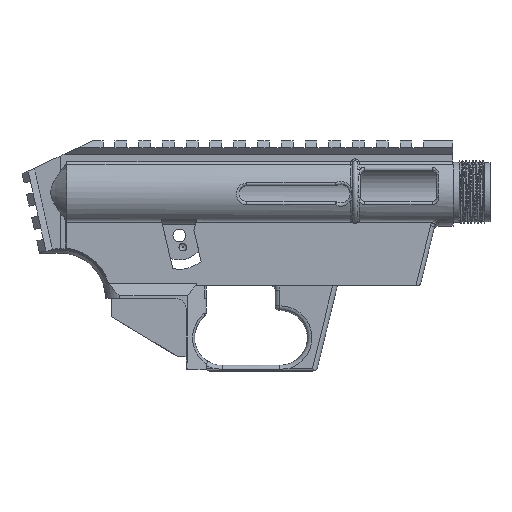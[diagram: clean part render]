
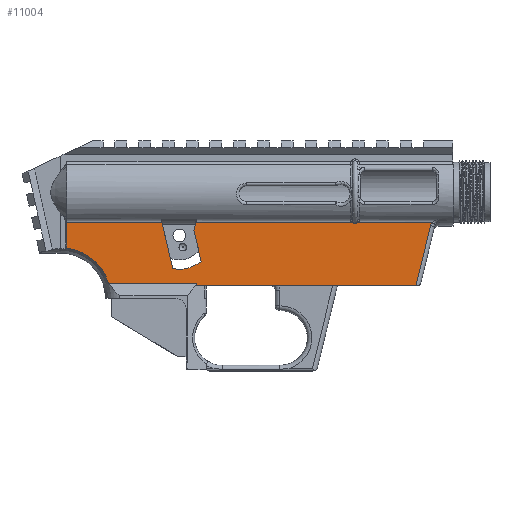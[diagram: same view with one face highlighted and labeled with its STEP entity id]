
A CAD part, left-side view. The second image highlights one B-rep face of the part: STEP entity #11004.
In plain terms, the highlighted planar face has unit normal (-1, 0, 0).
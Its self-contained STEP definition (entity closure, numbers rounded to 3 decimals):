
#329=B_SPLINE_CURVE_WITH_KNOTS('',3,(#16165,#16166,#16167,#16168,#16169,
#16170),.UNSPECIFIED.,.F.,.F.,(4,2,4),(0.,0.074,0.148),
 .UNSPECIFIED.);
#394=B_SPLINE_CURVE_WITH_KNOTS('',3,(#18997,#18998,#18999,#19000,#19001,
#19002,#19003,#19004,#19005,#19006,#19007,#19008),.UNSPECIFIED.,.F.,.F.,
(4,2,2,2,2,4),(0.,0.021,0.047,0.063,
0.077,0.097),.UNSPECIFIED.);
#395=B_SPLINE_CURVE_WITH_KNOTS('',3,(#19010,#19011,#19012,#19013,#19014,
#19015,#19016,#19017,#19018,#19019,#19020,#19021,#19022),.UNSPECIFIED.,
 .F.,.F.,(4,2,2,3,2,4),(-0.102,-0.09,-0.043,
0.,0.045,0.072),.UNSPECIFIED.);
#593=CIRCLE('',#11296,14.884);
#682=CIRCLE('',#11611,22.405);
#1240=FACE_OUTER_BOUND('',#1842,.T.);
#1842=EDGE_LOOP('',(#9356,#9357,#9358,#9359,#9360,#9361,#9362,#9363,#9364,
#9365,#9366,#9367,#9368,#9369,#9370,#9371));
#2151=LINE('',#15496,#3264);
#2157=LINE('',#15549,#3270);
#2257=LINE('',#15911,#3370);
#2300=LINE('',#16174,#3413);
#2599=LINE('',#16787,#3712);
#2652=LINE('',#17004,#3765);
#2696=LINE('',#17621,#3809);
#2697=LINE('',#17634,#3810);
#2920=LINE('',#18765,#4033);
#2932=LINE('',#18994,#4045);
#2933=LINE('',#19009,#4046);
#3264=VECTOR('',#12430,10.);
#3270=VECTOR('',#12458,10.);
#3370=VECTOR('',#12756,10.);
#3413=VECTOR('',#12895,10.);
#3712=VECTOR('',#13366,10.);
#3765=VECTOR('',#13485,10.);
#3809=VECTOR('',#13627,10.);
#3810=VECTOR('',#13634,10.);
#4033=VECTOR('',#14225,10.);
#4045=VECTOR('',#14267,10.);
#4046=VECTOR('',#14270,10.);
#4417=VERTEX_POINT('',#15494);
#4418=VERTEX_POINT('',#15495);
#4426=VERTEX_POINT('',#15547);
#4427=VERTEX_POINT('',#15548);
#4521=VERTEX_POINT('',#15905);
#4573=VERTEX_POINT('',#16162);
#4574=VERTEX_POINT('',#16164);
#4575=VERTEX_POINT('',#16173);
#4803=VERTEX_POINT('',#16785);
#4839=VERTEX_POINT('',#16999);
#4885=VERTEX_POINT('',#17618);
#4886=VERTEX_POINT('',#17620);
#4887=VERTEX_POINT('',#17633);
#5035=VERTEX_POINT('',#18760);
#5046=VERTEX_POINT('',#18843);
#5048=VERTEX_POINT('',#18996);
#5524=EDGE_CURVE('',#4417,#4418,#2151,.T.);
#5537=EDGE_CURVE('',#4426,#4427,#2157,.T.);
#5542=EDGE_CURVE('',#4418,#4426,#593,.T.);
#5685=EDGE_CURVE('',#4427,#4521,#2257,.T.);
#5758=EDGE_CURVE('',#4573,#4574,#329,.T.);
#5760=EDGE_CURVE('',#4574,#4575,#2300,.T.);
#6060=EDGE_CURVE('',#4803,#4417,#2599,.T.);
#6139=EDGE_CURVE('',#4839,#4803,#2652,.T.);
#6226=EDGE_CURVE('',#4886,#4885,#2696,.T.);
#6228=EDGE_CURVE('',#4886,#4839,#682,.T.);
#6229=EDGE_CURVE('',#4885,#4887,#2697,.T.);
#6527=EDGE_CURVE('',#5035,#4573,#2920,.T.);
#6553=EDGE_CURVE('',#4521,#5046,#2932,.T.);
#6554=EDGE_CURVE('',#5048,#5046,#394,.T.);
#6555=EDGE_CURVE('',#4575,#4887,#2933,.T.);
#6556=EDGE_CURVE('',#5035,#5048,#395,.T.);
#9356=ORIENTED_EDGE('',*,*,#6554,.T.);
#9357=ORIENTED_EDGE('',*,*,#6553,.F.);
#9358=ORIENTED_EDGE('',*,*,#5685,.F.);
#9359=ORIENTED_EDGE('',*,*,#5537,.F.);
#9360=ORIENTED_EDGE('',*,*,#5542,.F.);
#9361=ORIENTED_EDGE('',*,*,#5524,.F.);
#9362=ORIENTED_EDGE('',*,*,#6060,.F.);
#9363=ORIENTED_EDGE('',*,*,#6139,.F.);
#9364=ORIENTED_EDGE('',*,*,#6228,.F.);
#9365=ORIENTED_EDGE('',*,*,#6226,.T.);
#9366=ORIENTED_EDGE('',*,*,#6229,.T.);
#9367=ORIENTED_EDGE('',*,*,#6555,.F.);
#9368=ORIENTED_EDGE('',*,*,#5760,.F.);
#9369=ORIENTED_EDGE('',*,*,#5758,.F.);
#9370=ORIENTED_EDGE('',*,*,#6527,.F.);
#9371=ORIENTED_EDGE('',*,*,#6556,.T.);
#10492=PLANE('',#11812);
#11004=ADVANCED_FACE('',(#1240),#10492,.T.);
#11296=AXIS2_PLACEMENT_3D('',#15557,#12465,#12466);
#11611=AXIS2_PLACEMENT_3D('',#17631,#13630,#13631);
#11812=AXIS2_PLACEMENT_3D('',#18995,#14268,#14269);
#12430=DIRECTION('',(0.,-0.229,-0.973));
#12458=DIRECTION('',(0.,0.225,0.974));
#12465=DIRECTION('center_axis',(-1.,0.,0.));
#12466=DIRECTION('ref_axis',(0.,-1.,0.));
#12756=DIRECTION('',(0.,-0.225,0.974));
#12895=DIRECTION('',(0.,0.236,-0.972));
#13366=DIRECTION('',(0.,-1.,0.));
#13485=DIRECTION('',(0.,0.,1.));
#13627=DIRECTION('',(0.,-1.,0.));
#13630=DIRECTION('center_axis',(-1.,0.,0.));
#13631=DIRECTION('ref_axis',(0.,0.,1.));
#13634=DIRECTION('',(0.,0.,-1.));
#14225=DIRECTION('',(0.,-1.,0.));
#14267=DIRECTION('',(0.,-1.,0.));
#14268=DIRECTION('center_axis',(-1.,0.,0.));
#14269=DIRECTION('ref_axis',(0.,0.,1.));
#14270=DIRECTION('',(0.,1.,0.));
#15494=CARTESIAN_POINT('',(-8.42,50.391,27.845));
#15495=CARTESIAN_POINT('',(-8.42,45.62,7.575));
#15496=CARTESIAN_POINT('',(-8.42,43.577,-1.101));
#15547=CARTESIAN_POINT('',(-8.42,33.128,10.797));
#15548=CARTESIAN_POINT('',(-8.42,36.258,24.36));
#15549=CARTESIAN_POINT('',(-8.42,32.672,8.823));
#15557=CARTESIAN_POINT('Origin',(-8.42,42.724,22.175));
#15905=CARTESIAN_POINT('',(-8.42,35.445,27.888));
#15911=CARTESIAN_POINT('',(-8.42,37.307,19.808));
#16162=CARTESIAN_POINT('',(-8.42,-68.554,27.888));
#16164=CARTESIAN_POINT('',(-8.42,-67.981,26.535));
#16165=CARTESIAN_POINT('Ctrl Pts',(-8.42,-68.554,27.888));
#16166=CARTESIAN_POINT('Ctrl Pts',(-8.42,-68.423,27.68));
#16167=CARTESIAN_POINT('Ctrl Pts',(-8.42,-68.308,27.461));
#16168=CARTESIAN_POINT('Ctrl Pts',(-8.42,-68.116,27.008));
#16169=CARTESIAN_POINT('Ctrl Pts',(-8.42,-68.039,26.774));
#16170=CARTESIAN_POINT('Ctrl Pts',(-8.42,-67.981,26.535));
#16173=CARTESIAN_POINT('',(-8.42,-61.545,0.));
#16174=CARTESIAN_POINT('',(-8.42,-59.885,-6.843));
#16785=CARTESIAN_POINT('',(-8.42,92.25,27.845));
#16787=CARTESIAN_POINT('',(-8.42,0.,27.845));
#16999=CARTESIAN_POINT('',(-8.42,92.25,16.62));
#17004=CARTESIAN_POINT('',(-8.42,92.25,27.235));
#17618=CARTESIAN_POINT('',(-8.42,34.978,0.971));
#17620=CARTESIAN_POINT('',(-8.42,73.825,0.971));
#17621=CARTESIAN_POINT('',(-8.42,29.708,0.971));
#17631=CARTESIAN_POINT('Origin',(-8.42,95.25,-5.583));
#17633=CARTESIAN_POINT('',(-8.42,34.978,0.));
#17634=CARTESIAN_POINT('',(-8.42,34.978,0.));
#18760=CARTESIAN_POINT('',(-8.42,-35.664,27.888));
#18765=CARTESIAN_POINT('',(-8.42,0.,27.888));
#18843=CARTESIAN_POINT('',(-8.42,-33.329,27.888));
#18994=CARTESIAN_POINT('',(-8.42,0.,27.888));
#18995=CARTESIAN_POINT('Origin',(-8.42,0.,0.));
#18996=CARTESIAN_POINT('',(-8.42,-34.046,27.659));
#18997=CARTESIAN_POINT('Ctrl Pts',(-8.42,-34.046,27.659));
#18998=CARTESIAN_POINT('Ctrl Pts',(-8.42,-33.992,27.704));
#18999=CARTESIAN_POINT('Ctrl Pts',(-8.42,-33.933,27.741));
#19000=CARTESIAN_POINT('Ctrl Pts',(-8.42,-33.793,27.81));
#19001=CARTESIAN_POINT('Ctrl Pts',(-8.42,-33.722,27.831));
#19002=CARTESIAN_POINT('Ctrl Pts',(-8.42,-33.629,27.852));
#19003=CARTESIAN_POINT('Ctrl Pts',(-8.42,-33.594,27.859));
#19004=CARTESIAN_POINT('Ctrl Pts',(-8.42,-33.527,27.868));
#19005=CARTESIAN_POINT('Ctrl Pts',(-8.42,-33.495,27.872));
#19006=CARTESIAN_POINT('Ctrl Pts',(-8.42,-33.419,27.88));
#19007=CARTESIAN_POINT('Ctrl Pts',(-8.42,-33.377,27.884));
#19008=CARTESIAN_POINT('Ctrl Pts',(-8.42,-33.329,27.888));
#19009=CARTESIAN_POINT('',(-8.42,17.489,0.));
#19010=CARTESIAN_POINT('Ctrl Pts',(-8.42,-35.664,27.888));
#19011=CARTESIAN_POINT('Ctrl Pts',(-8.42,-35.638,27.853));
#19012=CARTESIAN_POINT('Ctrl Pts',(-8.42,-35.61,27.819));
#19013=CARTESIAN_POINT('Ctrl Pts',(-8.42,-35.478,27.674));
#19014=CARTESIAN_POINT('Ctrl Pts',(-8.42,-35.329,27.561));
#19015=CARTESIAN_POINT('Ctrl Pts',(-8.42,-35.057,27.438));
#19016=CARTESIAN_POINT('Ctrl Pts',(-8.42,-34.889,27.401));
#19017=CARTESIAN_POINT('Ctrl Pts',(-8.42,-34.746,27.401));
#19018=CARTESIAN_POINT('Ctrl Pts',(-8.42,-34.597,27.401));
#19019=CARTESIAN_POINT('Ctrl Pts',(-8.42,-34.422,27.442));
#19020=CARTESIAN_POINT('Ctrl Pts',(-8.42,-34.206,27.544));
#19021=CARTESIAN_POINT('Ctrl Pts',(-8.42,-34.122,27.597));
#19022=CARTESIAN_POINT('Ctrl Pts',(-8.42,-34.046,27.659));
